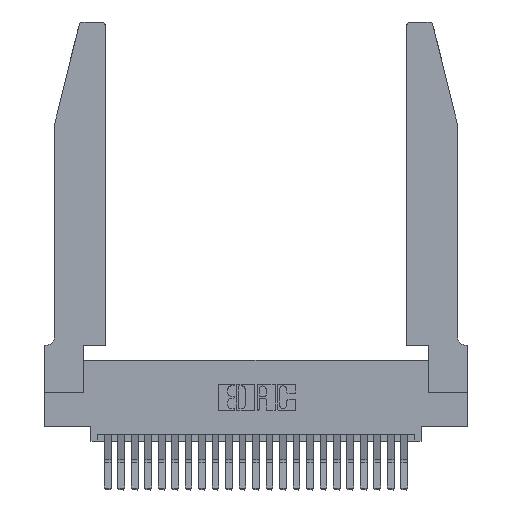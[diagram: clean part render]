
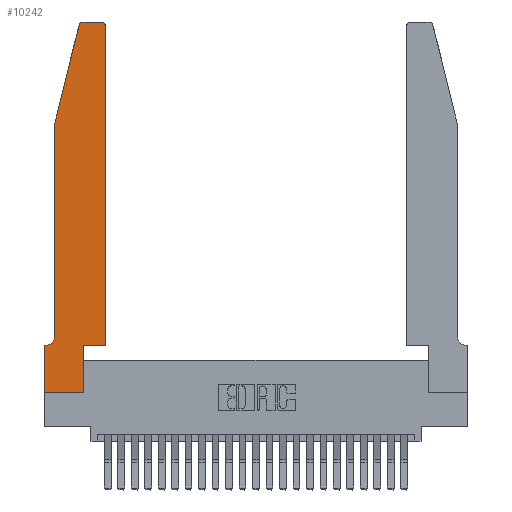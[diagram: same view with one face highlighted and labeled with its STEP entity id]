
A CAD part, top view. The second image highlights one B-rep face of the part: STEP entity #10242.
In plain terms, the highlighted planar face has unit normal (0, 0, 1).
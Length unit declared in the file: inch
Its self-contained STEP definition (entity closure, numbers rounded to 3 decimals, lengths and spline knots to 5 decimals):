
#262 = DIRECTION ( 'NONE',  ( 0., -1., 0. ) ) ;
#663 = PLANE ( 'NONE',  #22914 ) ;
#753 = EDGE_CURVE ( 'NONE', #11560, #7755, #4791, .T. ) ;
#1073 = CARTESIAN_POINT ( 'NONE',  ( 0.0755, 2., 0.37 ) ) ;
#1410 = LINE ( 'NONE', #15635, #11580 ) ;
#1545 = LINE ( 'NONE', #9885, #19107 ) ;
#1614 = CARTESIAN_POINT ( 'NONE',  ( 0.25487, 2.72718, 0.37 ) ) ;
#1912 = EDGE_CURVE ( 'NONE', #23347, #18803, #24235, .T. ) ;
#2425 = LINE ( 'NONE', #23747, #14415 ) ;
#2444 = LINE ( 'NONE', #16542, #12637 ) ;
#2800 = DIRECTION ( 'NONE',  ( 0., 0., 1. ) ) ;
#2990 = CARTESIAN_POINT ( 'NONE',  ( 0.4205, 2.75, 0.37 ) ) ;
#3290 = ORIENTED_EDGE ( 'NONE', *, *, #24356, .T. ) ;
#3479 = LINE ( 'NONE', #9934, #6887 ) ;
#3542 = DIRECTION ( 'NONE',  ( 0., 0., 1. ) ) ;
#3543 = DIRECTION ( 'NONE',  ( 0., -1., 0. ) ) ;
#4006 = CARTESIAN_POINT ( 'NONE',  ( 0.0055, 0.42, 0.37 ) ) ;
#4791 = LINE ( 'NONE', #12409, #16509 ) ;
#4838 = DIRECTION ( 'NONE',  ( 1., 0., 0. ) ) ;
#5468 = VERTEX_POINT ( 'NONE', #11269 ) ;
#5705 = AXIS2_PLACEMENT_3D ( 'NONE', #9423, #2800, #4838 ) ;
#6088 = DIRECTION ( 'NONE',  ( 0., 1., 0. ) ) ;
#6628 = DIRECTION ( 'NONE',  ( 0., 0., 1. ) ) ;
#6887 = VECTOR ( 'NONE', #262, 39.37008 ) ;
#6991 = VERTEX_POINT ( 'NONE', #20269 ) ;
#7071 = ORIENTED_EDGE ( 'NONE', *, *, #16552, .T. ) ;
#7755 = VERTEX_POINT ( 'NONE', #24256 ) ;
#8501 = DIRECTION ( 'NONE',  ( -0.239, -0.971, 0. ) ) ;
#8617 = EDGE_CURVE ( 'NONE', #18803, #13915, #3479, .T. ) ;
#8632 = DIRECTION ( 'NONE',  ( 1., 0., 0. ) ) ;
#9193 = VERTEX_POINT ( 'NONE', #18706 ) ;
#9411 = CARTESIAN_POINT ( 'NONE',  ( 0.284, 2.72, 0.37 ) ) ;
#9423 = CARTESIAN_POINT ( 'NONE',  ( 0.4205, 2.72, 0.37 ) ) ;
#9885 = CARTESIAN_POINT ( 'NONE',  ( 0.2865, 0.35, 0.37 ) ) ;
#9903 = DIRECTION ( 'NONE',  ( 1., 0., 0. ) ) ;
#9934 = CARTESIAN_POINT ( 'NONE',  ( 0.0755, 2., 0.37 ) ) ;
#9959 = EDGE_CURVE ( 'NONE', #7755, #23347, #22584, .T. ) ;
#10050 = VECTOR ( 'NONE', #8501, 39.37008 ) ;
#10091 = AXIS2_PLACEMENT_3D ( 'NONE', #4006, #13902, #21805 ) ;
#10242 = ADVANCED_FACE ( 'NONE', ( #14485 ), #663, .T. ) ;
#10385 = EDGE_CURVE ( 'NONE', #22785, #11560, #15705, .T. ) ;
#10520 = DIRECTION ( 'NONE',  ( -1., 0., 0. ) ) ;
#10775 = ORIENTED_EDGE ( 'NONE', *, *, #18175, .T. ) ;
#11017 = EDGE_CURVE ( 'NONE', #5468, #18801, #1545, .T. ) ;
#11269 = CARTESIAN_POINT ( 'NONE',  ( 0.2865, 0., 0.37 ) ) ;
#11560 = VERTEX_POINT ( 'NONE', #2990 ) ;
#11580 = VECTOR ( 'NONE', #3543, 39.37008 ) ;
#11929 = DIRECTION ( 'NONE',  ( -1., 0., 0. ) ) ;
#12409 = CARTESIAN_POINT ( 'NONE',  ( 0.2605, 2.75, 0.37 ) ) ;
#12472 = CIRCLE ( 'NONE', #10091, 0.07 ) ;
#12637 = VECTOR ( 'NONE', #8632, 39.37008 ) ;
#13251 = DIRECTION ( 'NONE',  ( 0., 1., 0. ) ) ;
#13902 = DIRECTION ( 'NONE',  ( 0., 0., -1. ) ) ;
#13915 = VERTEX_POINT ( 'NONE', #22920 ) ;
#14148 = ORIENTED_EDGE ( 'NONE', *, *, #11017, .T. ) ;
#14350 = DIRECTION ( 'NONE',  ( 1., 0., 0. ) ) ;
#14415 = VECTOR ( 'NONE', #11929, 39.37008 ) ;
#14485 = FACE_OUTER_BOUND ( 'NONE', #19551, .T. ) ;
#14702 = DIRECTION ( 'NONE',  ( 1., 0., 0. ) ) ;
#14786 = ORIENTED_EDGE ( 'NONE', *, *, #8617, .T. ) ;
#14850 = CARTESIAN_POINT ( 'NONE',  ( 0.4505, 2.72, 0.37 ) ) ;
#15235 = EDGE_CURVE ( 'NONE', #6991, #9193, #1410, .T. ) ;
#15635 = CARTESIAN_POINT ( 'NONE',  ( 0., 0., 0.37 ) ) ;
#15705 = CIRCLE ( 'NONE', #5705, 0.03 ) ;
#16059 = CARTESIAN_POINT ( 'NONE',  ( 0.0055, 0.35, 0.37 ) ) ;
#16241 = CARTESIAN_POINT ( 'NONE',  ( 0., 0.35, 0.37 ) ) ;
#16509 = VECTOR ( 'NONE', #10520, 39.37008 ) ;
#16520 = LINE ( 'NONE', #22496, #18710 ) ;
#16542 = CARTESIAN_POINT ( 'NONE',  ( 0., 0., 0.37 ) ) ;
#16552 = EDGE_CURVE ( 'NONE', #22503, #22785, #21129, .T. ) ;
#16710 = EDGE_CURVE ( 'NONE', #13915, #22086, #12472, .T. ) ;
#17172 = ORIENTED_EDGE ( 'NONE', *, *, #25338, .T. ) ;
#17218 = ORIENTED_EDGE ( 'NONE', *, *, #16710, .T. ) ;
#17672 = ORIENTED_EDGE ( 'NONE', *, *, #753, .T. ) ;
#18175 = EDGE_CURVE ( 'NONE', #18801, #22503, #16520, .T. ) ;
#18706 = CARTESIAN_POINT ( 'NONE',  ( 0., 0., 0.37 ) ) ;
#18710 = VECTOR ( 'NONE', #14702, 39.37008 ) ;
#18801 = VERTEX_POINT ( 'NONE', #20727 ) ;
#18803 = VERTEX_POINT ( 'NONE', #1073 ) ;
#18953 = CARTESIAN_POINT ( 'NONE',  ( 0.4505, 0.35, 0.37 ) ) ;
#19107 = VECTOR ( 'NONE', #6088, 39.37008 ) ;
#19453 = ORIENTED_EDGE ( 'NONE', *, *, #10385, .T. ) ;
#19551 = EDGE_LOOP ( 'NONE', ( #17672, #20780, #20895, #14786, #17218, #17172, #20957, #3290, #14148, #10775, #7071, #19453 ) ) ;
#20249 = AXIS2_PLACEMENT_3D ( 'NONE', #9411, #3542, #9903 ) ;
#20269 = CARTESIAN_POINT ( 'NONE',  ( 0., 0.35, 0.37 ) ) ;
#20727 = CARTESIAN_POINT ( 'NONE',  ( 0.2865, 0.35, 0.37 ) ) ;
#20780 = ORIENTED_EDGE ( 'NONE', *, *, #9959, .T. ) ;
#20895 = ORIENTED_EDGE ( 'NONE', *, *, #1912, .T. ) ;
#20957 = ORIENTED_EDGE ( 'NONE', *, *, #15235, .T. ) ;
#21129 = LINE ( 'NONE', #18953, #22987 ) ;
#21805 = DIRECTION ( 'NONE',  ( -1., 0., 0. ) ) ;
#22086 = VERTEX_POINT ( 'NONE', #16059 ) ;
#22496 = CARTESIAN_POINT ( 'NONE',  ( 0.4505, 0.35, 0.37 ) ) ;
#22503 = VERTEX_POINT ( 'NONE', #25450 ) ;
#22584 = CIRCLE ( 'NONE', #20249, 0.03 ) ;
#22785 = VERTEX_POINT ( 'NONE', #14850 ) ;
#22914 = AXIS2_PLACEMENT_3D ( 'NONE', #16241, #6628, #14350 ) ;
#22920 = CARTESIAN_POINT ( 'NONE',  ( 0.0755, 0.42, 0.37 ) ) ;
#22987 = VECTOR ( 'NONE', #13251, 39.37008 ) ;
#23347 = VERTEX_POINT ( 'NONE', #1614 ) ;
#23668 = CARTESIAN_POINT ( 'NONE',  ( 0.0755, 2., 0.37 ) ) ;
#23747 = CARTESIAN_POINT ( 'NONE',  ( 0.0755, 0.35, 0.37 ) ) ;
#24235 = LINE ( 'NONE', #23668, #10050 ) ;
#24256 = CARTESIAN_POINT ( 'NONE',  ( 0.284, 2.75, 0.37 ) ) ;
#24356 = EDGE_CURVE ( 'NONE', #9193, #5468, #2444, .T. ) ;
#25338 = EDGE_CURVE ( 'NONE', #22086, #6991, #2425, .T. ) ;
#25450 = CARTESIAN_POINT ( 'NONE',  ( 0.4505, 0.35, 0.37 ) ) ;
